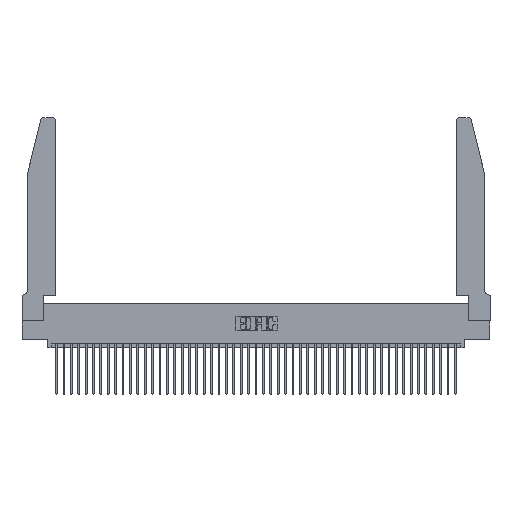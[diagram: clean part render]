
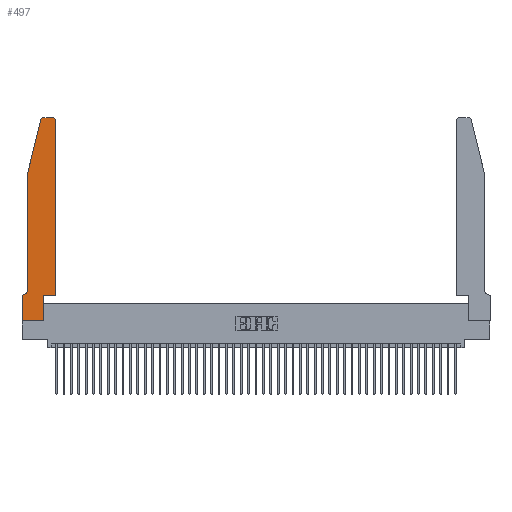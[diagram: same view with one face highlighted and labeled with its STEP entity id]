
A CAD part, top view. The second image highlights one B-rep face of the part: STEP entity #497.
In plain terms, the highlighted planar face has unit normal (0, 0, 1).
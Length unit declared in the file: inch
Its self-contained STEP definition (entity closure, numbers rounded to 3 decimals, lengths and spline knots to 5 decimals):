
#497 = ADVANCED_FACE ( 'NONE', ( #1220 ), #13208, .T. ) ;
#1118 = VERTEX_POINT ( 'NONE', #23773 ) ;
#1220 = FACE_OUTER_BOUND ( 'NONE', #43918, .T. ) ;
#1589 = DIRECTION ( 'NONE',  ( -1., 0., 0. ) ) ;
#3272 = LINE ( 'NONE', #37786, #33017 ) ;
#3389 = ORIENTED_EDGE ( 'NONE', *, *, #45189, .T. ) ;
#4041 = VECTOR ( 'NONE', #19602, 39.37008 ) ;
#4248 = VECTOR ( 'NONE', #34147, 39.37008 ) ;
#4417 = CARTESIAN_POINT ( 'NONE',  ( 0.4205, 2.72, 0.37 ) ) ;
#4441 = CARTESIAN_POINT ( 'NONE',  ( 0.284, 2.72, 0.37 ) ) ;
#5080 = LINE ( 'NONE', #27662, #12472 ) ;
#5132 = CARTESIAN_POINT ( 'NONE',  ( 0.0755, 0.35, 0.37 ) ) ;
#5134 = ORIENTED_EDGE ( 'NONE', *, *, #11283, .T. ) ;
#5505 = CARTESIAN_POINT ( 'NONE',  ( 0.2605, 2.75, 0.37 ) ) ;
#5642 = VERTEX_POINT ( 'NONE', #44833 ) ;
#5721 = CARTESIAN_POINT ( 'NONE',  ( 0.0755, 2., 0.37 ) ) ;
#5893 = LINE ( 'NONE', #5132, #33320 ) ;
#7129 = EDGE_CURVE ( 'NONE', #7677, #24920, #9651, .T. ) ;
#7677 = VERTEX_POINT ( 'NONE', #34243 ) ;
#8116 = DIRECTION ( 'NONE',  ( 1., 0., 0. ) ) ;
#8150 = DIRECTION ( 'NONE',  ( 1., 0., 0. ) ) ;
#8475 = VECTOR ( 'NONE', #10308, 39.37008 ) ;
#8563 = ORIENTED_EDGE ( 'NONE', *, *, #11948, .T. ) ;
#9077 = VECTOR ( 'NONE', #13601, 39.37008 ) ;
#9651 = LINE ( 'NONE', #38616, #8475 ) ;
#9956 = ORIENTED_EDGE ( 'NONE', *, *, #23929, .T. ) ;
#10308 = DIRECTION ( 'NONE',  ( 1., 0., 0. ) ) ;
#10315 = VERTEX_POINT ( 'NONE', #37831 ) ;
#10945 = AXIS2_PLACEMENT_3D ( 'NONE', #4417, #29525, #8116 ) ;
#11207 = CIRCLE ( 'NONE', #27277, 0.03 ) ;
#11283 = EDGE_CURVE ( 'NONE', #1118, #5642, #11207, .T. ) ;
#11948 = EDGE_CURVE ( 'NONE', #22574, #1118, #12811, .T. ) ;
#12472 = VECTOR ( 'NONE', #41884, 39.37008 ) ;
#12811 = LINE ( 'NONE', #5505, #4248 ) ;
#12913 = EDGE_CURVE ( 'NONE', #15966, #10315, #29437, .T. ) ;
#13208 = PLANE ( 'NONE',  #40332 ) ;
#13601 = DIRECTION ( 'NONE',  ( 0., 1., 0. ) ) ;
#13735 = LINE ( 'NONE', #26628, #4041 ) ;
#14028 = CARTESIAN_POINT ( 'NONE',  ( 0.2865, 0.35, 0.37 ) ) ;
#14295 = ORIENTED_EDGE ( 'NONE', *, *, #42462, .T. ) ;
#15966 = VERTEX_POINT ( 'NONE', #30148 ) ;
#16800 = DIRECTION ( 'NONE',  ( 0., 0., 1. ) ) ;
#16884 = CARTESIAN_POINT ( 'NONE',  ( 0.4205, 2.75, 0.37 ) ) ;
#18293 = CARTESIAN_POINT ( 'NONE',  ( 0.4505, 2.72, 0.37 ) ) ;
#18367 = LINE ( 'NONE', #14028, #36125 ) ;
#18389 = EDGE_CURVE ( 'NONE', #21868, #22402, #13735, .T. ) ;
#18615 = LINE ( 'NONE', #31360, #9077 ) ;
#18647 = VERTEX_POINT ( 'NONE', #31570 ) ;
#19602 = DIRECTION ( 'NONE',  ( 0., -1., 0. ) ) ;
#19974 = VECTOR ( 'NONE', #28962, 39.37008 ) ;
#20095 = DIRECTION ( 'NONE',  ( 1., 0., 0. ) ) ;
#20317 = VERTEX_POINT ( 'NONE', #29561 ) ;
#20723 = ORIENTED_EDGE ( 'NONE', *, *, #12913, .T. ) ;
#21343 = AXIS2_PLACEMENT_3D ( 'NONE', #44426, #23198, #1589 ) ;
#21868 = VERTEX_POINT ( 'NONE', #5721 ) ;
#22233 = ORIENTED_EDGE ( 'NONE', *, *, #23031, .T. ) ;
#22402 = VERTEX_POINT ( 'NONE', #26705 ) ;
#22574 = VERTEX_POINT ( 'NONE', #16884 ) ;
#22728 = ORIENTED_EDGE ( 'NONE', *, *, #18389, .T. ) ;
#23031 = EDGE_CURVE ( 'NONE', #10315, #20317, #3272, .T. ) ;
#23198 = DIRECTION ( 'NONE',  ( 0., 0., -1. ) ) ;
#23773 = CARTESIAN_POINT ( 'NONE',  ( 0.284, 2.75, 0.37 ) ) ;
#23929 = EDGE_CURVE ( 'NONE', #22402, #18647, #34035, .T. ) ;
#24815 = DIRECTION ( 'NONE',  ( 0., 1., 0. ) ) ;
#24920 = VERTEX_POINT ( 'NONE', #39084 ) ;
#26167 = ORIENTED_EDGE ( 'NONE', *, *, #7129, .T. ) ;
#26581 = EDGE_CURVE ( 'NONE', #5642, #21868, #5080, .T. ) ;
#26628 = CARTESIAN_POINT ( 'NONE',  ( 0.0755, 2., 0.37 ) ) ;
#26705 = CARTESIAN_POINT ( 'NONE',  ( 0.0755, 0.42, 0.37 ) ) ;
#27277 = AXIS2_PLACEMENT_3D ( 'NONE', #4441, #29554, #8150 ) ;
#27662 = CARTESIAN_POINT ( 'NONE',  ( 0.0755, 2., 0.37 ) ) ;
#28962 = DIRECTION ( 'NONE',  ( 0., -1., 0. ) ) ;
#29130 = ORIENTED_EDGE ( 'NONE', *, *, #32348, .T. ) ;
#29437 = LINE ( 'NONE', #32382, #19974 ) ;
#29525 = DIRECTION ( 'NONE',  ( 0., 0., 1. ) ) ;
#29554 = DIRECTION ( 'NONE',  ( 0., 0., 1. ) ) ;
#29561 = CARTESIAN_POINT ( 'NONE',  ( 0.2865, 0., 0.37 ) ) ;
#30148 = CARTESIAN_POINT ( 'NONE',  ( 0., 0.35, 0.37 ) ) ;
#30324 = CIRCLE ( 'NONE', #10945, 0.03 ) ;
#31360 = CARTESIAN_POINT ( 'NONE',  ( 0.4505, 0.35, 0.37 ) ) ;
#31570 = CARTESIAN_POINT ( 'NONE',  ( 0.0055, 0.35, 0.37 ) ) ;
#32348 = EDGE_CURVE ( 'NONE', #36657, #22574, #30324, .T. ) ;
#32382 = CARTESIAN_POINT ( 'NONE',  ( 0., 0., 0.37 ) ) ;
#33017 = VECTOR ( 'NONE', #20095, 39.37008 ) ;
#33320 = VECTOR ( 'NONE', #33788, 39.37008 ) ;
#33788 = DIRECTION ( 'NONE',  ( -1., 0., 0. ) ) ;
#34035 = CIRCLE ( 'NONE', #21343, 0.07 ) ;
#34147 = DIRECTION ( 'NONE',  ( -1., 0., 0. ) ) ;
#34243 = CARTESIAN_POINT ( 'NONE',  ( 0.2865, 0.35, 0.37 ) ) ;
#35430 = ORIENTED_EDGE ( 'NONE', *, *, #37201, .T. ) ;
#36125 = VECTOR ( 'NONE', #24815, 39.37008 ) ;
#36657 = VERTEX_POINT ( 'NONE', #18293 ) ;
#37201 = EDGE_CURVE ( 'NONE', #20317, #7677, #18367, .T. ) ;
#37786 = CARTESIAN_POINT ( 'NONE',  ( 0., 0., 0.37 ) ) ;
#37831 = CARTESIAN_POINT ( 'NONE',  ( 0., 0., 0.37 ) ) ;
#38072 = CARTESIAN_POINT ( 'NONE',  ( 0., 0.35, 0.37 ) ) ;
#38616 = CARTESIAN_POINT ( 'NONE',  ( 0.4505, 0.35, 0.37 ) ) ;
#39084 = CARTESIAN_POINT ( 'NONE',  ( 0.4505, 0.35, 0.37 ) ) ;
#40332 = AXIS2_PLACEMENT_3D ( 'NONE', #38072, #16800, #41639 ) ;
#41639 = DIRECTION ( 'NONE',  ( 1., 0., 0. ) ) ;
#41884 = DIRECTION ( 'NONE',  ( -0.239, -0.971, 0. ) ) ;
#42278 = ORIENTED_EDGE ( 'NONE', *, *, #26581, .T. ) ;
#42462 = EDGE_CURVE ( 'NONE', #18647, #15966, #5893, .T. ) ;
#43918 = EDGE_LOOP ( 'NONE', ( #8563, #5134, #42278, #22728, #9956, #14295, #20723, #22233, #35430, #26167, #3389, #29130 ) ) ;
#44426 = CARTESIAN_POINT ( 'NONE',  ( 0.0055, 0.42, 0.37 ) ) ;
#44833 = CARTESIAN_POINT ( 'NONE',  ( 0.25487, 2.72718, 0.37 ) ) ;
#45189 = EDGE_CURVE ( 'NONE', #24920, #36657, #18615, .T. ) ;
